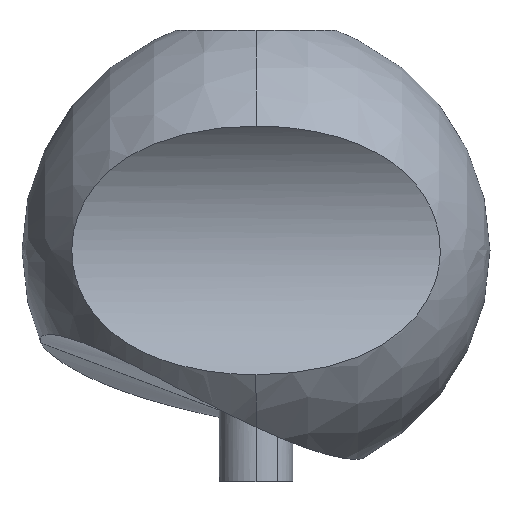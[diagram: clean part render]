
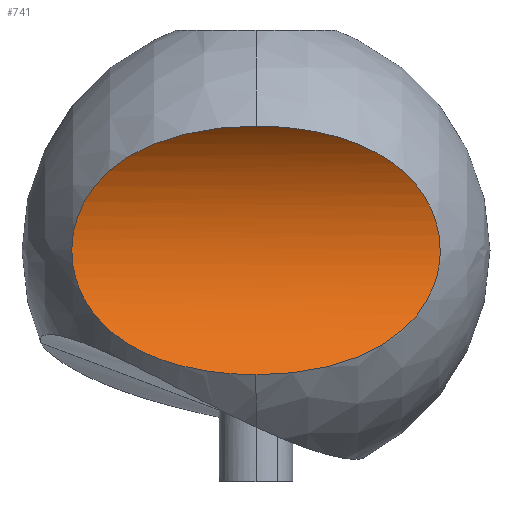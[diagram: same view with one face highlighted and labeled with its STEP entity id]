
A CAD part, left-side view. The second image highlights one B-rep face of the part: STEP entity #741.
In plain terms, the highlighted cylindrical face has radius 8 mm (diameter 16 mm), a partial arc.
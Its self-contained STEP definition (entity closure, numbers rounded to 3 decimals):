
#9 = B_SPLINE_CURVE_WITH_KNOTS ( 'NONE', 3,
 ( #124, #123, #122, #121, #120, #119, #118, #117, #116, #115, #114, #113, #112, #111, #110, #109, #108, #107, #106, #105, #104, #103, #102, #101, #100, #99, #98, #94, #95, #96, #91, #92, #93, #88, #89, #90, #85, #84, #83, #82 ),
 .UNSPECIFIED., .F., .F.,
 ( 4, 2, 2, 2, 2, 2, 2, 2, 2, 2, 2, 2, 2, 2, 2, 2, 2, 2, 2, 4 ),
 ( 0.024, 0.025, 0.027, 0.028, 0.03, 0.031, 0.032, 0.033, 0.034, 0.035, 0.035, 0.036, 0.037, 0.038, 0.04, 0.041, 0.043, 0.044, 0.046, 0.047 ),
 .UNSPECIFIED. ) ;
#22 = B_SPLINE_CURVE_WITH_KNOTS ( 'NONE', 3,
 ( #203, #202, #201, #200, #199, #198, #197, #196, #195, #194, #193, #192, #191, #190, #189, #188, #187, #186, #185, #184, #183, #182, #181, #180, #179, #178, #177, #176, #175, #174, #173, #172, #171, #170, #169, #168, #167, #166, #165, #164, #163, #162 ),
 .UNSPECIFIED., .F., .F.,
 ( 4, 2, 2, 2, 2, 2, 2, 2, 2, 2, 2, 2, 2, 2, 2, 2, 2, 2, 2, 2, 4 ),
 ( 0., 0.003, 0.004, 0.004, 0.006, 0.007, 0.007, 0.009, 0.01, 0.012, 0.013, 0.013, 0.015, 0.016, 0.017, 0.018, 0.019, 0.02, 0.021, 0.022, 0.024 ),
 .UNSPECIFIED. ) ;
#82 = CARTESIAN_POINT ( 'NONE',  ( -9.32, 0., -5.843 ) ) ;
#83 = CARTESIAN_POINT ( 'NONE',  ( -9.32, 0.5, -5.843 ) ) ;
#84 = CARTESIAN_POINT ( 'NONE',  ( -9.294, 0.998, -5.82 ) ) ;
#85 = CARTESIAN_POINT ( 'NONE',  ( -9.195, 1.984, -5.724 ) ) ;
#88 = CARTESIAN_POINT ( 'NONE',  ( -8.812, 3.901, -5.327 ) ) ;
#89 = CARTESIAN_POINT ( 'NONE',  ( -8.928, 3.435, -5.453 ) ) ;
#90 = CARTESIAN_POINT ( 'NONE',  ( -9.12, 2.474, -5.652 ) ) ;
#91 = CARTESIAN_POINT ( 'NONE',  ( -8.078, 6.075, -4.371 ) ) ;
#92 = CARTESIAN_POINT ( 'NONE',  ( -8.397, 5.239, -4.826 ) ) ;
#93 = CARTESIAN_POINT ( 'NONE',  ( -8.547, 4.802, -5.014 ) ) ;
#94 = CARTESIAN_POINT ( 'NONE',  ( -7.417, 7.505, -3.147 ) ) ;
#95 = CARTESIAN_POINT ( 'NONE',  ( -7.582, 7.178, -3.5 ) ) ;
#96 = CARTESIAN_POINT ( 'NONE',  ( -7.911, 6.464, -4.109 ) ) ;
#98 = CARTESIAN_POINT ( 'NONE',  ( -7.129, 8.053, -2.362 ) ) ;
#99 = CARTESIAN_POINT ( 'NONE',  ( -7.003, 8.277, -1.921 ) ) ;
#100 = CARTESIAN_POINT ( 'NONE',  ( -6.874, 8.504, -1.22 ) ) ;
#101 = CARTESIAN_POINT ( 'NONE',  ( -6.84, 8.563, -0.977 ) ) ;
#102 = CARTESIAN_POINT ( 'NONE',  ( -6.795, 8.641, -0.482 ) ) ;
#103 = CARTESIAN_POINT ( 'NONE',  ( -6.783, 8.66, -0.234 ) ) ;
#104 = CARTESIAN_POINT ( 'NONE',  ( -6.784, 8.658, 0.264 ) ) ;
#105 = CARTESIAN_POINT ( 'NONE',  ( -6.797, 8.637, 0.516 ) ) ;
#106 = CARTESIAN_POINT ( 'NONE',  ( -6.844, 8.556, 1.009 ) ) ;
#107 = CARTESIAN_POINT ( 'NONE',  ( -6.878, 8.496, 1.249 ) ) ;
#108 = CARTESIAN_POINT ( 'NONE',  ( -6.966, 8.342, 1.715 ) ) ;
#109 = CARTESIAN_POINT ( 'NONE',  ( -7.02, 8.247, 1.943 ) ) ;
#110 = CARTESIAN_POINT ( 'NONE',  ( -7.142, 8.026, 2.377 ) ) ;
#111 = CARTESIAN_POINT ( 'NONE',  ( -7.209, 7.901, 2.582 ) ) ;
#112 = CARTESIAN_POINT ( 'NONE',  ( -7.425, 7.489, 3.166 ) ) ;
#113 = CARTESIAN_POINT ( 'NONE',  ( -7.59, 7.161, 3.517 ) ) ;
#114 = CARTESIAN_POINT ( 'NONE',  ( -7.92, 6.444, 4.123 ) ) ;
#115 = CARTESIAN_POINT ( 'NONE',  ( -8.086, 6.054, 4.384 ) ) ;
#116 = CARTESIAN_POINT ( 'NONE',  ( -8.405, 5.216, 4.837 ) ) ;
#117 = CARTESIAN_POINT ( 'NONE',  ( -8.554, 4.78, 5.023 ) ) ;
#118 = CARTESIAN_POINT ( 'NONE',  ( -8.817, 3.882, 5.333 ) ) ;
#119 = CARTESIAN_POINT ( 'NONE',  ( -8.932, 3.418, 5.457 ) ) ;
#120 = CARTESIAN_POINT ( 'NONE',  ( -9.122, 2.464, 5.653 ) ) ;
#121 = CARTESIAN_POINT ( 'NONE',  ( -9.196, 1.971, 5.726 ) ) ;
#122 = CARTESIAN_POINT ( 'NONE',  ( -9.295, 0.988, 5.82 ) ) ;
#123 = CARTESIAN_POINT ( 'NONE',  ( -9.32, 0.495, 5.843 ) ) ;
#124 = CARTESIAN_POINT ( 'NONE',  ( -9.32, 0., 5.843 ) ) ;
#162 = CARTESIAN_POINT ( 'NONE',  ( -9.32, 0., 5.843 ) ) ;
#163 = CARTESIAN_POINT ( 'NONE',  ( -9.32, -0.496, 5.843 ) ) ;
#164 = CARTESIAN_POINT ( 'NONE',  ( -9.294, -0.996, 5.82 ) ) ;
#165 = CARTESIAN_POINT ( 'NONE',  ( -9.195, -1.986, 5.724 ) ) ;
#166 = CARTESIAN_POINT ( 'NONE',  ( -9.121, -2.473, 5.652 ) ) ;
#167 = CARTESIAN_POINT ( 'NONE',  ( -8.978, -3.189, 5.504 ) ) ;
#168 = CARTESIAN_POINT ( 'NONE',  ( -8.925, -3.426, 5.448 ) ) ;
#169 = CARTESIAN_POINT ( 'NONE',  ( -8.808, -3.895, 5.32 ) ) ;
#170 = CARTESIAN_POINT ( 'NONE',  ( -8.745, -4.128, 5.248 ) ) ;
#171 = CARTESIAN_POINT ( 'NONE',  ( -8.544, -4.809, 5.011 ) ) ;
#172 = CARTESIAN_POINT ( 'NONE',  ( -8.395, -5.244, 4.823 ) ) ;
#173 = CARTESIAN_POINT ( 'NONE',  ( -8.158, -5.864, 4.485 ) ) ;
#174 = CARTESIAN_POINT ( 'NONE',  ( -8.077, -6.065, 4.364 ) ) ;
#175 = CARTESIAN_POINT ( 'NONE',  ( -7.911, -6.456, 4.098 ) ) ;
#176 = CARTESIAN_POINT ( 'NONE',  ( -7.827, -6.646, 3.954 ) ) ;
#177 = CARTESIAN_POINT ( 'NONE',  ( -7.579, -7.182, 3.495 ) ) ;
#178 = CARTESIAN_POINT ( 'NONE',  ( -7.418, -7.503, 3.151 ) ) ;
#179 = CARTESIAN_POINT ( 'NONE',  ( -7.128, -8.055, 2.359 ) ) ;
#180 = CARTESIAN_POINT ( 'NONE',  ( -7.004, -8.276, 1.924 ) ) ;
#181 = CARTESIAN_POINT ( 'NONE',  ( -6.873, -8.506, 1.216 ) ) ;
#182 = CARTESIAN_POINT ( 'NONE',  ( -6.84, -8.563, 0.975 ) ) ;
#183 = CARTESIAN_POINT ( 'NONE',  ( -6.795, -8.641, 0.484 ) ) ;
#184 = CARTESIAN_POINT ( 'NONE',  ( -6.783, -8.66, 0.232 ) ) ;
#185 = CARTESIAN_POINT ( 'NONE',  ( -6.785, -8.657, -0.522 ) ) ;
#186 = CARTESIAN_POINT ( 'NONE',  ( -6.834, -8.575, -1.011 ) ) ;
#187 = CARTESIAN_POINT ( 'NONE',  ( -7.011, -8.263, -1.953 ) ) ;
#188 = CARTESIAN_POINT ( 'NONE',  ( -7.135, -8.042, -2.382 ) ) ;
#189 = CARTESIAN_POINT ( 'NONE',  ( -7.427, -7.486, -3.17 ) ) ;
#190 = CARTESIAN_POINT ( 'NONE',  ( -7.589, -7.163, -3.514 ) ) ;
#191 = CARTESIAN_POINT ( 'NONE',  ( -7.836, -6.625, -3.97 ) ) ;
#192 = CARTESIAN_POINT ( 'NONE',  ( -7.921, -6.435, -4.113 ) ) ;
#193 = CARTESIAN_POINT ( 'NONE',  ( -8.086, -6.043, -4.377 ) ) ;
#194 = CARTESIAN_POINT ( 'NONE',  ( -8.167, -5.841, -4.499 ) ) ;
#195 = CARTESIAN_POINT ( 'NONE',  ( -8.404, -5.22, -4.834 ) ) ;
#196 = CARTESIAN_POINT ( 'NONE',  ( -8.552, -4.785, -5.021 ) ) ;
#197 = CARTESIAN_POINT ( 'NONE',  ( -8.752, -4.103, -5.256 ) ) ;
#198 = CARTESIAN_POINT ( 'NONE',  ( -8.815, -3.87, -5.327 ) ) ;
#199 = CARTESIAN_POINT ( 'NONE',  ( -8.93, -3.401, -5.454 ) ) ;
#200 = CARTESIAN_POINT ( 'NONE',  ( -8.983, -3.166, -5.509 ) ) ;
#201 = CARTESIAN_POINT ( 'NONE',  ( -9.218, -1.978, -5.753 ) ) ;
#202 = CARTESIAN_POINT ( 'NONE',  ( -9.32, -1.002, -5.843 ) ) ;
#203 = CARTESIAN_POINT ( 'NONE',  ( -9.32, 0., -5.843 ) ) ;
#357 = DIRECTION ( 'NONE',  ( 0., 0., -1. ) ) ;
#358 = DIRECTION ( 'NONE',  ( 0., -1., 0. ) ) ;
#359 = CARTESIAN_POINT ( 'NONE',  ( -14.784, 11., 0. ) ) ;
#403 = CARTESIAN_POINT ( 'NONE',  ( -9.32, 0., 5.843 ) ) ;
#404 = CARTESIAN_POINT ( 'NONE',  ( -9.32, 0., -5.843 ) ) ;
#527 = EDGE_LOOP ( 'NONE', ( #623, #624 ) ) ;
#556 = VERTEX_POINT ( 'NONE', #404 ) ;
#557 = VERTEX_POINT ( 'NONE', #403 ) ;
#623 = ORIENTED_EDGE ( 'NONE', *, *, #767, .T. ) ;
#624 = ORIENTED_EDGE ( 'NONE', *, *, #770, .T. ) ;
#656 = CYLINDRICAL_SURFACE ( 'NONE', #657, 8. ) ;
#657 = AXIS2_PLACEMENT_3D ( 'NONE', #359, #358, #357 ) ;
#662 = FACE_OUTER_BOUND ( 'NONE', #527, .T. ) ;
#741 = ADVANCED_FACE ( 'NONE', ( #662 ), #656, .F. ) ;
#767 = EDGE_CURVE ( 'NONE', #556, #557, #22, .T. ) ;
#770 = EDGE_CURVE ( 'NONE', #557, #556, #9, .T. ) ;
